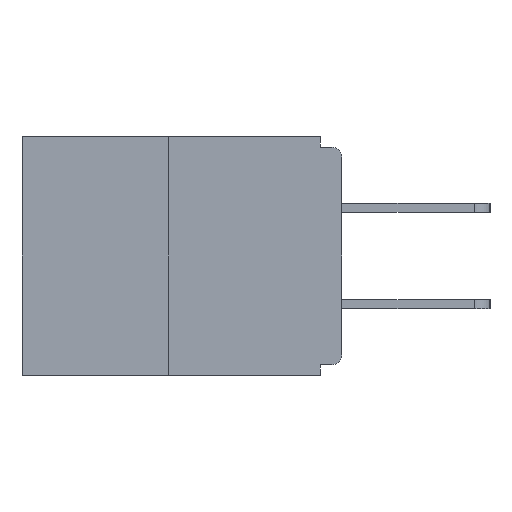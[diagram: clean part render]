
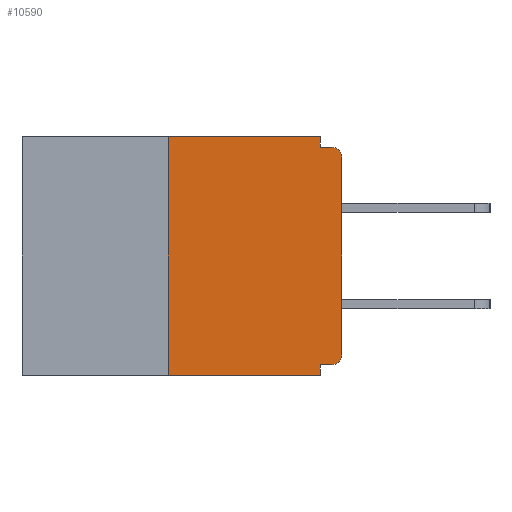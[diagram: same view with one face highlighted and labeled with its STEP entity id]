
A CAD part, left-side view. The second image highlights one B-rep face of the part: STEP entity #10590.
In plain terms, the highlighted planar face has unit normal (-1, 0, 0).
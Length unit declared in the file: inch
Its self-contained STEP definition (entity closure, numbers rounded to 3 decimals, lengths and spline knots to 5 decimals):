
#23 = DIRECTION ( 'NONE',  ( 0., 0., -1. ) ) ;
#270 = CARTESIAN_POINT ( 'NONE',  ( 0., 0., -0.313 ) ) ;
#453 = DIRECTION ( 'NONE',  ( 0., 0., 1. ) ) ;
#526 = ORIENTED_EDGE ( 'NONE', *, *, #6441, .T. ) ;
#544 = CARTESIAN_POINT ( 'NONE',  ( 0., 0.46, -0.343 ) ) ;
#547 = EDGE_CURVE ( 'NONE', #3642, #1486, #2291, .T. ) ;
#962 = VECTOR ( 'NONE', #9977, 39.37008 ) ;
#966 = EDGE_CURVE ( 'NONE', #7297, #1486, #6061, .T. ) ;
#1044 = EDGE_CURVE ( 'NONE', #3770, #3560, #8442, .T. ) ;
#1138 = VECTOR ( 'NONE', #4006, 39.37008 ) ;
#1207 = ORIENTED_EDGE ( 'NONE', *, *, #547, .F. ) ;
#1286 = EDGE_CURVE ( 'NONE', #8006, #3642, #9852, .T. ) ;
#1295 = DIRECTION ( 'NONE',  ( 0., 1., 0. ) ) ;
#1475 = CARTESIAN_POINT ( 'NONE',  ( 0., 0.015, -0.015 ) ) ;
#1486 = VERTEX_POINT ( 'NONE', #8489 ) ;
#1526 = ORIENTED_EDGE ( 'NONE', *, *, #8769, .F. ) ;
#1886 = CARTESIAN_POINT ( 'NONE',  ( 0., 0.015, -0.328 ) ) ;
#1967 = CARTESIAN_POINT ( 'NONE',  ( 0., 0.015, -0.03 ) ) ;
#2152 = CARTESIAN_POINT ( 'NONE',  ( 0., 0., -0.328 ) ) ;
#2158 = LINE ( 'NONE', #4762, #6398 ) ;
#2226 = DIRECTION ( 'NONE',  ( 0., 0., -1. ) ) ;
#2291 = LINE ( 'NONE', #5846, #3816 ) ;
#2318 = ORIENTED_EDGE ( 'NONE', *, *, #1286, .F. ) ;
#2323 = AXIS2_PLACEMENT_3D ( 'NONE', #6520, #6465, #2226 ) ;
#2446 = VECTOR ( 'NONE', #3292, 39.37008 ) ;
#2750 = PLANE ( 'NONE',  #5937 ) ;
#3167 = ORIENTED_EDGE ( 'NONE', *, *, #6898, .F. ) ;
#3292 = DIRECTION ( 'NONE',  ( 0., -1., 0. ) ) ;
#3339 = VECTOR ( 'NONE', #10117, 39.37008 ) ;
#3393 = CARTESIAN_POINT ( 'NONE',  ( 0., 0., -0.015 ) ) ;
#3488 = VERTEX_POINT ( 'NONE', #10306 ) ;
#3560 = VERTEX_POINT ( 'NONE', #3582 ) ;
#3582 = CARTESIAN_POINT ( 'NONE',  ( 0., 0.031, 0. ) ) ;
#3642 = VERTEX_POINT ( 'NONE', #7126 ) ;
#3668 = VERTEX_POINT ( 'NONE', #5438 ) ;
#3770 = VERTEX_POINT ( 'NONE', #10015 ) ;
#3788 = DIRECTION ( 'NONE',  ( 0., 0., -1. ) ) ;
#3816 = VECTOR ( 'NONE', #6638, 39.37008 ) ;
#4006 = DIRECTION ( 'NONE',  ( 0., 0., -1. ) ) ;
#4143 = DIRECTION ( 'NONE',  ( 0., -1., 0. ) ) ;
#4233 = EDGE_CURVE ( 'NONE', #3560, #3668, #4909, .T. ) ;
#4762 = CARTESIAN_POINT ( 'NONE',  ( 0., 0.25, 0. ) ) ;
#4803 = CARTESIAN_POINT ( 'NONE',  ( 0., 0.031, 0. ) ) ;
#4909 = LINE ( 'NONE', #4803, #1138 ) ;
#4973 = LINE ( 'NONE', #3393, #3339 ) ;
#4994 = CARTESIAN_POINT ( 'NONE',  ( 0., 0.46, 0. ) ) ;
#5349 = EDGE_CURVE ( 'NONE', #3488, #8327, #10415, .T. ) ;
#5381 = VERTEX_POINT ( 'NONE', #270 ) ;
#5438 = CARTESIAN_POINT ( 'NONE',  ( 0., 0.031, -0.015 ) ) ;
#5531 = AXIS2_PLACEMENT_3D ( 'NONE', #1967, #10749, #3788 ) ;
#5746 = ORIENTED_EDGE ( 'NONE', *, *, #1044, .F. ) ;
#5846 = CARTESIAN_POINT ( 'NONE',  ( 0., 0.031, -0.343 ) ) ;
#5937 = AXIS2_PLACEMENT_3D ( 'NONE', #6924, #8000, #23 ) ;
#6061 = LINE ( 'NONE', #544, #8407 ) ;
#6398 = VECTOR ( 'NONE', #453, 39.37008 ) ;
#6441 = EDGE_CURVE ( 'NONE', #5381, #3488, #8230, .T. ) ;
#6465 = DIRECTION ( 'NONE',  ( -1., 0., 0. ) ) ;
#6520 = CARTESIAN_POINT ( 'NONE',  ( 0., 0.015, -0.313 ) ) ;
#6638 = DIRECTION ( 'NONE',  ( 0., 0., -1. ) ) ;
#6898 = EDGE_CURVE ( 'NONE', #7297, #3770, #2158, .T. ) ;
#6924 = CARTESIAN_POINT ( 'NONE',  ( 0., 0.46, 0. ) ) ;
#7126 = CARTESIAN_POINT ( 'NONE',  ( 0., 0.031, -0.328 ) ) ;
#7297 = VERTEX_POINT ( 'NONE', #9161 ) ;
#7691 = EDGE_LOOP ( 'NONE', ( #5746, #3167, #9935, #1207, #2318, #8137, #526, #9323, #1526, #9491 ) ) ;
#7780 = FACE_OUTER_BOUND ( 'NONE', #7691, .T. ) ;
#8000 = DIRECTION ( 'NONE',  ( 1., 0., 0. ) ) ;
#8006 = VERTEX_POINT ( 'NONE', #1886 ) ;
#8137 = ORIENTED_EDGE ( 'NONE', *, *, #10611, .T. ) ;
#8230 = LINE ( 'NONE', #10828, #962 ) ;
#8327 = VERTEX_POINT ( 'NONE', #1475 ) ;
#8407 = VECTOR ( 'NONE', #4143, 39.37008 ) ;
#8442 = LINE ( 'NONE', #4994, #2446 ) ;
#8489 = CARTESIAN_POINT ( 'NONE',  ( 0., 0.031, -0.343 ) ) ;
#8769 = EDGE_CURVE ( 'NONE', #3668, #8327, #4973, .T. ) ;
#9161 = CARTESIAN_POINT ( 'NONE',  ( 0., 0.25, -0.343 ) ) ;
#9323 = ORIENTED_EDGE ( 'NONE', *, *, #5349, .T. ) ;
#9491 = ORIENTED_EDGE ( 'NONE', *, *, #4233, .F. ) ;
#9852 = LINE ( 'NONE', #2152, #10241 ) ;
#9935 = ORIENTED_EDGE ( 'NONE', *, *, #966, .T. ) ;
#9977 = DIRECTION ( 'NONE',  ( 0., 0., 1. ) ) ;
#10015 = CARTESIAN_POINT ( 'NONE',  ( 0., 0.25, 0. ) ) ;
#10117 = DIRECTION ( 'NONE',  ( 0., -1., 0. ) ) ;
#10241 = VECTOR ( 'NONE', #1295, 39.37008 ) ;
#10281 = CIRCLE ( 'NONE', #2323, 0.015 ) ;
#10306 = CARTESIAN_POINT ( 'NONE',  ( 0., 0., -0.03 ) ) ;
#10415 = CIRCLE ( 'NONE', #5531, 0.015 ) ;
#10590 = ADVANCED_FACE ( 'NONE', ( #7780 ), #2750, .F. ) ;
#10611 = EDGE_CURVE ( 'NONE', #8006, #5381, #10281, .T. ) ;
#10749 = DIRECTION ( 'NONE',  ( -1., 0., 0. ) ) ;
#10828 = CARTESIAN_POINT ( 'NONE',  ( 0., 0., 0. ) ) ;
